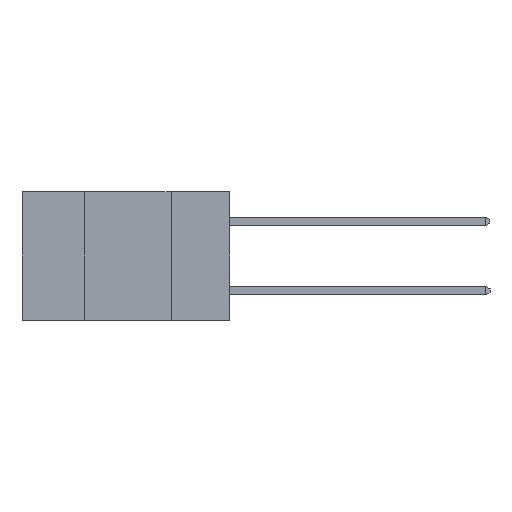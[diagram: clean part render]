
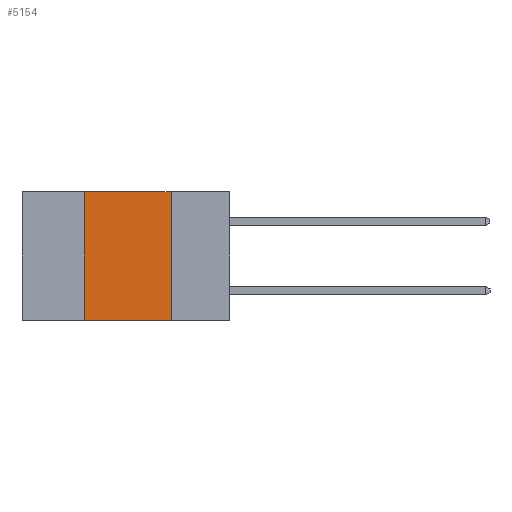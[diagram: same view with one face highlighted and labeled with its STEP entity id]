
A CAD part, left-side view. The second image highlights one B-rep face of the part: STEP entity #5154.
In plain terms, the highlighted planar face has unit normal (-1, 0, 0).
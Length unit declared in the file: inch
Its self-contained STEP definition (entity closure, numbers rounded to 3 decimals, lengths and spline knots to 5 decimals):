
#113 = ORIENTED_EDGE ( 'NONE', *, *, #1871, .F. ) ;
#233 = DIRECTION ( 'NONE',  ( 0., 0., -1. ) ) ;
#417 = VECTOR ( 'NONE', #233, 39.37008 ) ;
#572 = AXIS2_PLACEMENT_3D ( 'NONE', #3232, #4809, #7172 ) ;
#1332 = CARTESIAN_POINT ( 'NONE',  ( 0., 0.42, 0. ) ) ;
#1492 = ORIENTED_EDGE ( 'NONE', *, *, #7491, .T. ) ;
#1528 = PLANE ( 'NONE',  #572 ) ;
#1866 = CARTESIAN_POINT ( 'NONE',  ( 0., 0.42, -0.37 ) ) ;
#1871 = EDGE_CURVE ( 'NONE', #7308, #9164, #6108, .T. ) ;
#2309 = CARTESIAN_POINT ( 'NONE',  ( 0., 0.42, -0.37 ) ) ;
#2463 = EDGE_LOOP ( 'NONE', ( #10015, #2650, #113, #1492 ) ) ;
#2509 = LINE ( 'NONE', #9649, #417 ) ;
#2650 = ORIENTED_EDGE ( 'NONE', *, *, #5621, .F. ) ;
#2659 = VERTEX_POINT ( 'NONE', #9544 ) ;
#2825 = EDGE_CURVE ( 'NONE', #2659, #8422, #2509, .T. ) ;
#2870 = CARTESIAN_POINT ( 'NONE',  ( 0., 0.6, 0. ) ) ;
#3098 = LINE ( 'NONE', #5541, #7593 ) ;
#3232 = CARTESIAN_POINT ( 'NONE',  ( 0., 0.6, 0. ) ) ;
#3502 = VECTOR ( 'NONE', #4421, 39.37008 ) ;
#4421 = DIRECTION ( 'NONE',  ( 0., -1., 0. ) ) ;
#4489 = VECTOR ( 'NONE', #9352, 39.37008 ) ;
#4809 = DIRECTION ( 'NONE',  ( 1., 0., 0. ) ) ;
#5154 = ADVANCED_FACE ( 'NONE', ( #8026 ), #1528, .F. ) ;
#5541 = CARTESIAN_POINT ( 'NONE',  ( 0., 0.6, -0.37 ) ) ;
#5621 = EDGE_CURVE ( 'NONE', #9164, #2659, #9096, .T. ) ;
#6108 = LINE ( 'NONE', #2309, #4489 ) ;
#7045 = CARTESIAN_POINT ( 'NONE',  ( 0., 0.17, -0.37 ) ) ;
#7172 = DIRECTION ( 'NONE',  ( 0., 0., -1. ) ) ;
#7308 = VERTEX_POINT ( 'NONE', #1866 ) ;
#7491 = EDGE_CURVE ( 'NONE', #7308, #8422, #3098, .T. ) ;
#7593 = VECTOR ( 'NONE', #8009, 39.37008 ) ;
#8009 = DIRECTION ( 'NONE',  ( 0., -1., 0. ) ) ;
#8026 = FACE_OUTER_BOUND ( 'NONE', #2463, .T. ) ;
#8422 = VERTEX_POINT ( 'NONE', #7045 ) ;
#9096 = LINE ( 'NONE', #2870, #3502 ) ;
#9164 = VERTEX_POINT ( 'NONE', #1332 ) ;
#9352 = DIRECTION ( 'NONE',  ( 0., 0., 1. ) ) ;
#9544 = CARTESIAN_POINT ( 'NONE',  ( 0., 0.17, 0. ) ) ;
#9649 = CARTESIAN_POINT ( 'NONE',  ( 0., 0.17, -0.37 ) ) ;
#10015 = ORIENTED_EDGE ( 'NONE', *, *, #2825, .F. ) ;
